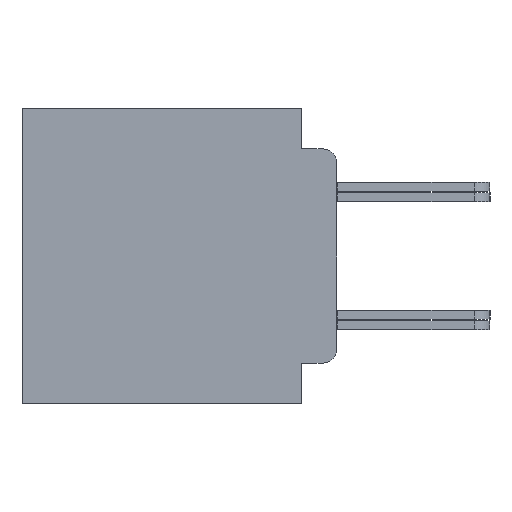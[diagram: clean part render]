
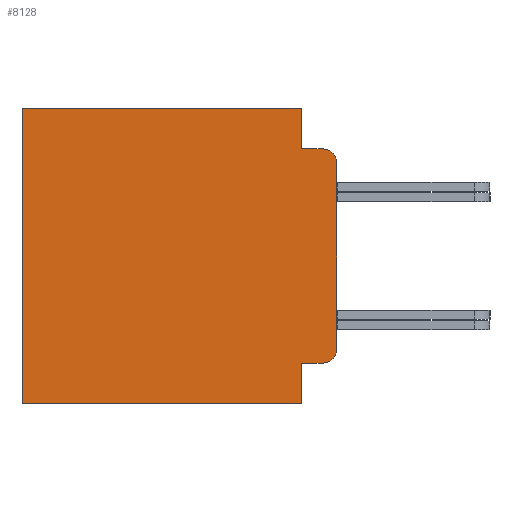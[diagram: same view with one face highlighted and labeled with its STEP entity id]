
A CAD part, left-side view. The second image highlights one B-rep face of the part: STEP entity #8128.
In plain terms, the highlighted planar face has unit normal (-1, 0, 0).
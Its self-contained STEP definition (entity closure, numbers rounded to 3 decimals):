
#90 = CARTESIAN_POINT ( 'NONE',  ( -67.462, 11.684, -5.486 ) ) ;
#189 = CARTESIAN_POINT ( 'NONE',  ( -67.462, 1.295, 0. ) ) ;
#370 = ORIENTED_EDGE ( 'NONE', *, *, #18229, .T. ) ;
#571 = AXIS2_PLACEMENT_3D ( 'NONE', #19192, #23608, #4139 ) ;
#856 = VECTOR ( 'NONE', #27440, 1000. ) ;
#1125 = LINE ( 'NONE', #27493, #22608 ) ;
#1226 = CARTESIAN_POINT ( 'NONE',  ( -67.462, 0., 5.486 ) ) ;
#1542 = LINE ( 'NONE', #3407, #856 ) ;
#1738 = VERTEX_POINT ( 'NONE', #11583 ) ;
#2087 = VERTEX_POINT ( 'NONE', #21841 ) ;
#2130 = EDGE_CURVE ( 'NONE', #24680, #2087, #13566, .T. ) ;
#3038 = EDGE_CURVE ( 'NONE', #14629, #17407, #1542, .T. ) ;
#3407 = CARTESIAN_POINT ( 'NONE',  ( -67.462, 1.295, 0. ) ) ;
#4139 = DIRECTION ( 'NONE',  ( 0., 0., -1. ) ) ;
#4240 = VECTOR ( 'NONE', #13858, 1000. ) ;
#4841 = EDGE_CURVE ( 'NONE', #14629, #11149, #1125, .T. ) ;
#5421 = VERTEX_POINT ( 'NONE', #20984 ) ;
#5483 = DIRECTION ( 'NONE',  ( 0., 1., 0. ) ) ;
#6683 = VECTOR ( 'NONE', #7733, 1000. ) ;
#6846 = ORIENTED_EDGE ( 'NONE', *, *, #22663, .F. ) ;
#7733 = DIRECTION ( 'NONE',  ( 0., 1., 0. ) ) ;
#7980 = CARTESIAN_POINT ( 'NONE',  ( -67.462, 0., -5.486 ) ) ;
#8128 = ADVANCED_FACE ( 'NONE', ( #10526 ), #23693, .F. ) ;
#9086 = CARTESIAN_POINT ( 'NONE',  ( -67.462, 0.508, -3.975 ) ) ;
#9239 = CARTESIAN_POINT ( 'NONE',  ( -67.462, 1.295, -5.486 ) ) ;
#9964 = VERTEX_POINT ( 'NONE', #26975 ) ;
#10139 = LINE ( 'NONE', #26970, #18954 ) ;
#10526 = FACE_OUTER_BOUND ( 'NONE', #13922, .T. ) ;
#11149 = VERTEX_POINT ( 'NONE', #9086 ) ;
#11550 = ORIENTED_EDGE ( 'NONE', *, *, #3038, .F. ) ;
#11583 = CARTESIAN_POINT ( 'NONE',  ( -67.462, 0., -3.467 ) ) ;
#12163 = LINE ( 'NONE', #1226, #6683 ) ;
#13566 = LINE ( 'NONE', #189, #23093 ) ;
#13567 = CARTESIAN_POINT ( 'NONE',  ( -67.462, 1.295, 5.486 ) ) ;
#13858 = DIRECTION ( 'NONE',  ( 0., -1., 0. ) ) ;
#13922 = EDGE_LOOP ( 'NONE', ( #14739, #16029, #15732, #370, #21202, #25079, #19132, #26996, #6846, #11550 ) ) ;
#14411 = DIRECTION ( 'NONE',  ( 0., -1., 0. ) ) ;
#14629 = VERTEX_POINT ( 'NONE', #25083 ) ;
#14739 = ORIENTED_EDGE ( 'NONE', *, *, #4841, .T. ) ;
#14910 = DIRECTION ( 'NONE',  ( 1., 0., 0. ) ) ;
#15553 = DIRECTION ( 'NONE',  ( 0., 0., -1. ) ) ;
#15732 = ORIENTED_EDGE ( 'NONE', *, *, #18582, .F. ) ;
#16006 = CARTESIAN_POINT ( 'NONE',  ( -67.462, 11.684, 5.486 ) ) ;
#16029 = ORIENTED_EDGE ( 'NONE', *, *, #16747, .T. ) ;
#16648 = CIRCLE ( 'NONE', #571, 0.508 ) ;
#16747 = EDGE_CURVE ( 'NONE', #11149, #1738, #19231, .T. ) ;
#17407 = VERTEX_POINT ( 'NONE', #9239 ) ;
#17785 = VECTOR ( 'NONE', #5483, 1000. ) ;
#17815 = DIRECTION ( 'NONE',  ( -1., 0., 0. ) ) ;
#18229 = EDGE_CURVE ( 'NONE', #5421, #9964, #16648, .T. ) ;
#18582 = EDGE_CURVE ( 'NONE', #5421, #1738, #20025, .T. ) ;
#18887 = LINE ( 'NONE', #20609, #4240 ) ;
#18954 = VECTOR ( 'NONE', #20260, 1000. ) ;
#19132 = ORIENTED_EDGE ( 'NONE', *, *, #24755, .T. ) ;
#19192 = CARTESIAN_POINT ( 'NONE',  ( -67.462, 0.508, 3.467 ) ) ;
#19231 = CIRCLE ( 'NONE', #23393, 0.508 ) ;
#19690 = VECTOR ( 'NONE', #23004, 1000. ) ;
#19789 = EDGE_CURVE ( 'NONE', #23899, #20792, #10139, .T. ) ;
#20025 = LINE ( 'NONE', #22907, #19690 ) ;
#20260 = DIRECTION ( 'NONE',  ( 0., 0., -1. ) ) ;
#20609 = CARTESIAN_POINT ( 'NONE',  ( -67.462, 1.295, 3.975 ) ) ;
#20792 = VERTEX_POINT ( 'NONE', #90 ) ;
#20984 = CARTESIAN_POINT ( 'NONE',  ( -67.462, 0., 3.467 ) ) ;
#21202 = ORIENTED_EDGE ( 'NONE', *, *, #26027, .F. ) ;
#21288 = CARTESIAN_POINT ( 'NONE',  ( -67.462, 0., -5.486 ) ) ;
#21841 = CARTESIAN_POINT ( 'NONE',  ( -67.462, 1.295, 3.975 ) ) ;
#22557 = LINE ( 'NONE', #7980, #17785 ) ;
#22608 = VECTOR ( 'NONE', #14411, 1000. ) ;
#22663 = EDGE_CURVE ( 'NONE', #17407, #20792, #22557, .T. ) ;
#22907 = CARTESIAN_POINT ( 'NONE',  ( -67.462, 0., -5.486 ) ) ;
#23004 = DIRECTION ( 'NONE',  ( 0., 0., -1. ) ) ;
#23093 = VECTOR ( 'NONE', #15553, 1000. ) ;
#23393 = AXIS2_PLACEMENT_3D ( 'NONE', #24517, #17815, #26434 ) ;
#23608 = DIRECTION ( 'NONE',  ( -1., 0., 0. ) ) ;
#23693 = PLANE ( 'NONE',  #26767 ) ;
#23899 = VERTEX_POINT ( 'NONE', #16006 ) ;
#24517 = CARTESIAN_POINT ( 'NONE',  ( -67.462, 0.508, -3.467 ) ) ;
#24680 = VERTEX_POINT ( 'NONE', #13567 ) ;
#24755 = EDGE_CURVE ( 'NONE', #24680, #23899, #12163, .T. ) ;
#25079 = ORIENTED_EDGE ( 'NONE', *, *, #2130, .F. ) ;
#25083 = CARTESIAN_POINT ( 'NONE',  ( -67.462, 1.295, -3.975 ) ) ;
#26027 = EDGE_CURVE ( 'NONE', #2087, #9964, #18887, .T. ) ;
#26434 = DIRECTION ( 'NONE',  ( 0., 0., -1. ) ) ;
#26767 = AXIS2_PLACEMENT_3D ( 'NONE', #21288, #14910, #28082 ) ;
#26970 = CARTESIAN_POINT ( 'NONE',  ( -67.462, 11.684, -5.486 ) ) ;
#26975 = CARTESIAN_POINT ( 'NONE',  ( -67.462, 0.508, 3.975 ) ) ;
#26996 = ORIENTED_EDGE ( 'NONE', *, *, #19789, .T. ) ;
#27440 = DIRECTION ( 'NONE',  ( 0., 0., -1. ) ) ;
#27493 = CARTESIAN_POINT ( 'NONE',  ( -67.462, 1.295, -3.975 ) ) ;
#28082 = DIRECTION ( 'NONE',  ( 0., 0., -1. ) ) ;
